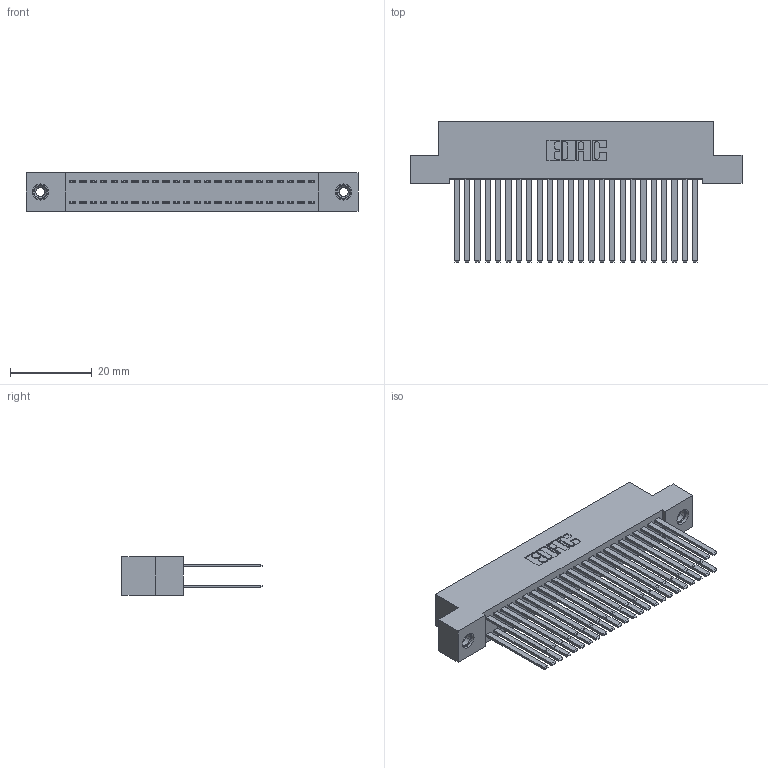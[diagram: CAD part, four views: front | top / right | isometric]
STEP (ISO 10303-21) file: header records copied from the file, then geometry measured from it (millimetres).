
FILE_DESCRIPTION (( 'STEP AP203' ), '1' );
FILE_NAME ('342-048-544-208.STEP', '2019-10-02T22:18:49', ( '' ), ( '' ), 'SwSTEP 2.0', 'SolidWorks 2016', '' );
FILE_SCHEMA (( 'CONFIG_CONTROL_DESIGN' ));
Length unit declared in the file: inch
Products named in the file (4): 342 Part_TI; 345-292-001_345-293-144; 345-250-001_345-250-003-102; 342-048-544-208
Assembly tree (51 placements, depth 2):
  342-048-544-208
    342 Part_TI
    345-292-001_345-293-144  x48
    345-250-001_345-250-003-102  x2
Bounding box: 81.28 x 34.3 x 9.4 mm (x, y, z)
Volume: 7885 mm3; surface area: 14264.9 mm2
Topology: 51 solids, 51 shells, 2378 faces, 7011 edges, 4602 vertices
Faces by surface type: plane 1634, cylinder 728, cone 12, torus 4
Entity records: 18638 total; most frequent: CARTESIAN_POINT 3089, ORIENTED_EDGE 3018, DIRECTION 2699, EDGE_CURVE 1509, LINE 1365, VECTOR 1365, VERTEX_POINT 1000, AXIS2_PLACEMENT_3D 667
